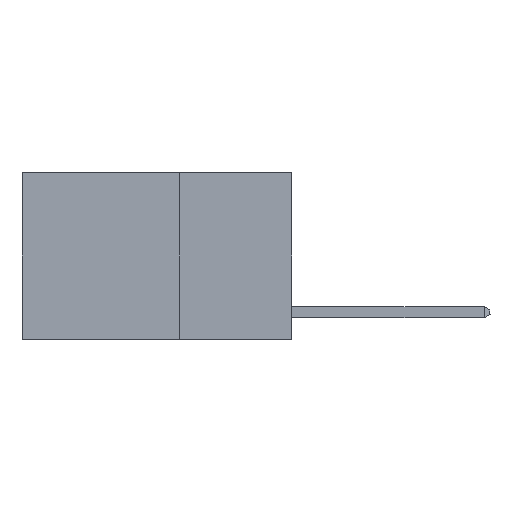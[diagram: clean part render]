
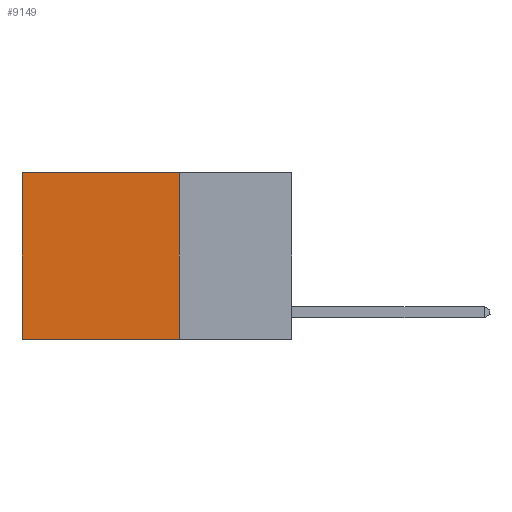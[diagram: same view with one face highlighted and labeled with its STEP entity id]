
A CAD part, left-side view. The second image highlights one B-rep face of the part: STEP entity #9149.
In plain terms, the highlighted planar face has unit normal (-1, 0, 0).
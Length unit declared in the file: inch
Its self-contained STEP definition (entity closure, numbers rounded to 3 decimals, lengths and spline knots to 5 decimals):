
#275 = VECTOR ( 'NONE', #20023, 39.37008 ) ;
#1364 = FACE_OUTER_BOUND ( 'NONE', #24275, .T. ) ;
#1592 = ORIENTED_EDGE ( 'NONE', *, *, #20439, .T. ) ;
#1779 = VERTEX_POINT ( 'NONE', #13600 ) ;
#3227 = CARTESIAN_POINT ( 'NONE',  ( 0.2625, 0.25, -0.37 ) ) ;
#3861 = ORIENTED_EDGE ( 'NONE', *, *, #26699, .T. ) ;
#4741 = DIRECTION ( 'NONE',  ( 1., 0., 0. ) ) ;
#5930 = LINE ( 'NONE', #3227, #275 ) ;
#5982 = DIRECTION ( 'NONE',  ( 0., 0., -1. ) ) ;
#7037 = DIRECTION ( 'NONE',  ( 0., 0., -1. ) ) ;
#7153 = VECTOR ( 'NONE', #5982, 39.37008 ) ;
#9149 = ADVANCED_FACE ( 'NONE', ( #1364 ), #15251, .F. ) ;
#9869 = ORIENTED_EDGE ( 'NONE', *, *, #16241, .F. ) ;
#10157 = CARTESIAN_POINT ( 'NONE',  ( 0.2625, 0.25, 0. ) ) ;
#11263 = ORIENTED_EDGE ( 'NONE', *, *, #19746, .F. ) ;
#11769 = VERTEX_POINT ( 'NONE', #26867 ) ;
#12757 = LINE ( 'NONE', #10157, #7153 ) ;
#13031 = AXIS2_PLACEMENT_3D ( 'NONE', #23584, #4741, #19458 ) ;
#13110 = VERTEX_POINT ( 'NONE', #20742 ) ;
#13399 = CARTESIAN_POINT ( 'NONE',  ( 0.2625, 0.6, 0. ) ) ;
#13600 = CARTESIAN_POINT ( 'NONE',  ( 0.2625, 0.25, -0.37 ) ) ;
#14051 = LINE ( 'NONE', #22097, #18930 ) ;
#15251 = PLANE ( 'NONE',  #13031 ) ;
#16241 = EDGE_CURVE ( 'NONE', #11769, #1779, #12757, .T. ) ;
#18930 = VECTOR ( 'NONE', #24232, 39.37008 ) ;
#19458 = DIRECTION ( 'NONE',  ( 0., 0., -1. ) ) ;
#19746 = EDGE_CURVE ( 'NONE', #1779, #13110, #5930, .T. ) ;
#19900 = CARTESIAN_POINT ( 'NONE',  ( 0.2625, 0.6, 0. ) ) ;
#20023 = DIRECTION ( 'NONE',  ( 0., 1., 0. ) ) ;
#20439 = EDGE_CURVE ( 'NONE', #11769, #24019, #14051, .T. ) ;
#20742 = CARTESIAN_POINT ( 'NONE',  ( 0.2625, 0.6, -0.37 ) ) ;
#22097 = CARTESIAN_POINT ( 'NONE',  ( 0.2625, 0.25, 0. ) ) ;
#23584 = CARTESIAN_POINT ( 'NONE',  ( 0.2625, 0.25, 0. ) ) ;
#24019 = VERTEX_POINT ( 'NONE', #19900 ) ;
#24232 = DIRECTION ( 'NONE',  ( 0., 1., 0. ) ) ;
#24275 = EDGE_LOOP ( 'NONE', ( #3861, #11263, #9869, #1592 ) ) ;
#24639 = VECTOR ( 'NONE', #7037, 39.37008 ) ;
#25259 = LINE ( 'NONE', #13399, #24639 ) ;
#26699 = EDGE_CURVE ( 'NONE', #24019, #13110, #25259, .T. ) ;
#26867 = CARTESIAN_POINT ( 'NONE',  ( 0.2625, 0.25, 0. ) ) ;
